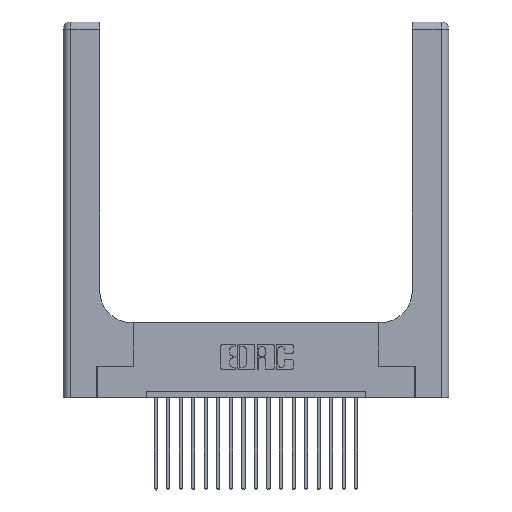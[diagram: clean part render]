
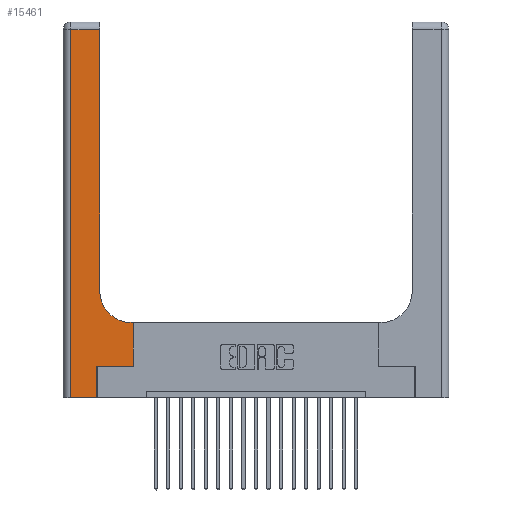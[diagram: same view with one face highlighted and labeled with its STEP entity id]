
A CAD part, top view. The second image highlights one B-rep face of the part: STEP entity #15461.
In plain terms, the highlighted planar face has unit normal (0, 0, 1).
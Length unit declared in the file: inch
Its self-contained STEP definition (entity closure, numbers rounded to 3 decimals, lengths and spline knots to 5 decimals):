
#19 = CARTESIAN_POINT ( 'NONE',  ( 0.5585, 0.6, 0.37 ) ) ;
#116 = DIRECTION ( 'NONE',  ( 0., -1., 0. ) ) ;
#388 = VERTEX_POINT ( 'NONE', #20344 ) ;
#1547 = LINE ( 'NONE', #11617, #14920 ) ;
#2137 = CARTESIAN_POINT ( 'NONE',  ( 0.06, 2.94, 0.37 ) ) ;
#2458 = EDGE_CURVE ( 'NONE', #388, #19767, #12288, .T. ) ;
#2496 = VERTEX_POINT ( 'NONE', #18992 ) ;
#2672 = LINE ( 'NONE', #8214, #19416 ) ;
#2695 = LINE ( 'NONE', #6662, #10357 ) ;
#3598 = CARTESIAN_POINT ( 'NONE',  ( 0.2915, 3., 0.37 ) ) ;
#4057 = CARTESIAN_POINT ( 'NONE',  ( 0.269, 0.25, 0.37 ) ) ;
#4293 = EDGE_CURVE ( 'NONE', #10180, #10264, #13002, .T. ) ;
#4511 = FACE_OUTER_BOUND ( 'NONE', #7743, .T. ) ;
#4574 = EDGE_CURVE ( 'NONE', #15869, #17625, #2695, .T. ) ;
#4779 = ORIENTED_EDGE ( 'NONE', *, *, #20318, .T. ) ;
#5199 = VECTOR ( 'NONE', #12511, 39.37008 ) ;
#5714 = DIRECTION ( 'NONE',  ( 1., 0., 0. ) ) ;
#5838 = CARTESIAN_POINT ( 'NONE',  ( 0.2915, 2.94, 0.37 ) ) ;
#6001 = CARTESIAN_POINT ( 'NONE',  ( 0., 0., 0.37 ) ) ;
#6346 = EDGE_CURVE ( 'NONE', #17625, #9213, #11612, .T. ) ;
#6662 = CARTESIAN_POINT ( 'NONE',  ( 0.06, 3., 0.37 ) ) ;
#6824 = DIRECTION ( 'NONE',  ( 0., 1., 0. ) ) ;
#7132 = EDGE_CURVE ( 'NONE', #10264, #15869, #1547, .T. ) ;
#7246 = CARTESIAN_POINT ( 'NONE',  ( 0.269, 0., 0.37 ) ) ;
#7525 = ORIENTED_EDGE ( 'NONE', *, *, #7132, .T. ) ;
#7743 = EDGE_LOOP ( 'NONE', ( #11983, #7525, #16134, #16421, #4779, #10876, #11055, #17496, #12321 ) ) ;
#8214 = CARTESIAN_POINT ( 'NONE',  ( 0.5585, 0.25, 0.37 ) ) ;
#9213 = VERTEX_POINT ( 'NONE', #7246 ) ;
#9741 = DIRECTION ( 'NONE',  ( 0., 1., 0. ) ) ;
#9781 = LINE ( 'NONE', #13027, #13428 ) ;
#9783 = DIRECTION ( 'NONE',  ( 1., 0., 0. ) ) ;
#9865 = VECTOR ( 'NONE', #10817, 39.37008 ) ;
#10067 = CARTESIAN_POINT ( 'NONE',  ( 0.06, 0., 0.37 ) ) ;
#10180 = VERTEX_POINT ( 'NONE', #10679 ) ;
#10264 = VERTEX_POINT ( 'NONE', #5838 ) ;
#10357 = VECTOR ( 'NONE', #116, 39.37008 ) ;
#10679 = CARTESIAN_POINT ( 'NONE',  ( 0.2915, 0.85, 0.37 ) ) ;
#10817 = DIRECTION ( 'NONE',  ( -1., 0., 0. ) ) ;
#10876 = ORIENTED_EDGE ( 'NONE', *, *, #2458, .T. ) ;
#11055 = ORIENTED_EDGE ( 'NONE', *, *, #16731, .T. ) ;
#11612 = LINE ( 'NONE', #6001, #5199 ) ;
#11617 = CARTESIAN_POINT ( 'NONE',  ( 0., 2.94, 0.37 ) ) ;
#11983 = ORIENTED_EDGE ( 'NONE', *, *, #4293, .T. ) ;
#12288 = LINE ( 'NONE', #4057, #13324 ) ;
#12321 = ORIENTED_EDGE ( 'NONE', *, *, #17945, .T. ) ;
#12427 = CARTESIAN_POINT ( 'NONE',  ( 0.2915, 0.6, 0.37 ) ) ;
#12511 = DIRECTION ( 'NONE',  ( 1., 0., 0. ) ) ;
#13002 = LINE ( 'NONE', #3598, #16099 ) ;
#13027 = CARTESIAN_POINT ( 'NONE',  ( 0.269, 0., 0.37 ) ) ;
#13209 = DIRECTION ( 'NONE',  ( 0., 0., -1. ) ) ;
#13324 = VECTOR ( 'NONE', #5714, 39.37008 ) ;
#13428 = VECTOR ( 'NONE', #9741, 39.37008 ) ;
#14276 = PLANE ( 'NONE',  #18518 ) ;
#14478 = VERTEX_POINT ( 'NONE', #19 ) ;
#14495 = DIRECTION ( 'NONE',  ( 0., 1., 0. ) ) ;
#14920 = VECTOR ( 'NONE', #16491, 39.37008 ) ;
#15461 = ADVANCED_FACE ( 'NONE', ( #4511 ), #14276, .F. ) ;
#15489 = EDGE_CURVE ( 'NONE', #14478, #2496, #16633, .T. ) ;
#15869 = VERTEX_POINT ( 'NONE', #2137 ) ;
#15937 = DIRECTION ( 'NONE',  ( -1., 0., 0. ) ) ;
#16099 = VECTOR ( 'NONE', #6824, 39.37008 ) ;
#16134 = ORIENTED_EDGE ( 'NONE', *, *, #4574, .T. ) ;
#16421 = ORIENTED_EDGE ( 'NONE', *, *, #6346, .T. ) ;
#16491 = DIRECTION ( 'NONE',  ( -1., 0., 0. ) ) ;
#16516 = CIRCLE ( 'NONE', #21161, 0.25 ) ;
#16633 = LINE ( 'NONE', #12427, #9865 ) ;
#16731 = EDGE_CURVE ( 'NONE', #19767, #14478, #2672, .T. ) ;
#17496 = ORIENTED_EDGE ( 'NONE', *, *, #15489, .T. ) ;
#17625 = VERTEX_POINT ( 'NONE', #10067 ) ;
#17945 = EDGE_CURVE ( 'NONE', #2496, #10180, #16516, .T. ) ;
#18064 = CARTESIAN_POINT ( 'NONE',  ( 0.5415, 0.85, 0.37 ) ) ;
#18518 = AXIS2_PLACEMENT_3D ( 'NONE', #20931, #21077, #15937 ) ;
#18992 = CARTESIAN_POINT ( 'NONE',  ( 0.5415, 0.6, 0.37 ) ) ;
#19416 = VECTOR ( 'NONE', #14495, 39.37008 ) ;
#19767 = VERTEX_POINT ( 'NONE', #19991 ) ;
#19991 = CARTESIAN_POINT ( 'NONE',  ( 0.5585, 0.25, 0.37 ) ) ;
#20318 = EDGE_CURVE ( 'NONE', #9213, #388, #9781, .T. ) ;
#20344 = CARTESIAN_POINT ( 'NONE',  ( 0.269, 0.25, 0.37 ) ) ;
#20931 = CARTESIAN_POINT ( 'NONE',  ( 0., 3., 0.37 ) ) ;
#21077 = DIRECTION ( 'NONE',  ( 0., 0., -1. ) ) ;
#21161 = AXIS2_PLACEMENT_3D ( 'NONE', #18064, #13209, #9783 ) ;
